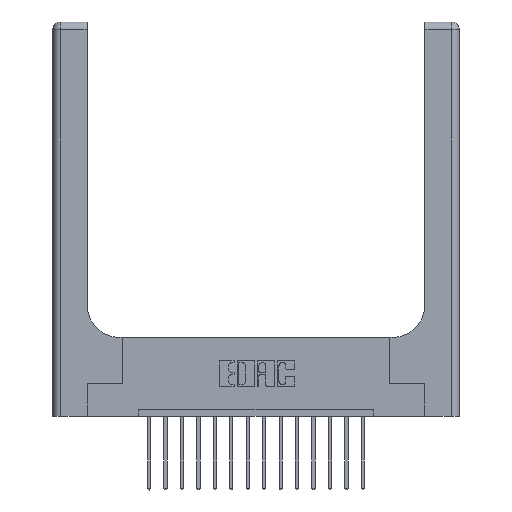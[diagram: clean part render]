
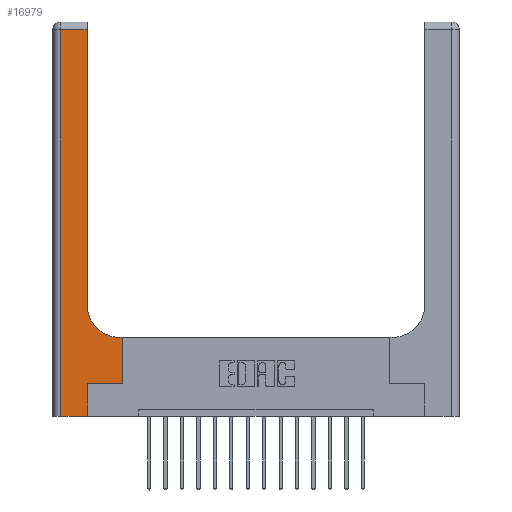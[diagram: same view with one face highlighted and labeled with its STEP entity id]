
A CAD part, top view. The second image highlights one B-rep face of the part: STEP entity #16979.
In plain terms, the highlighted planar face has unit normal (0, 0, 1).
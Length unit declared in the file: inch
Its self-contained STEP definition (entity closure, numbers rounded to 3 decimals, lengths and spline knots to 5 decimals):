
#4 = LINE ( 'NONE', #4893, #426 ) ;
#426 = VECTOR ( 'NONE', #14502, 39.37008 ) ;
#449 = VECTOR ( 'NONE', #7445, 39.37008 ) ;
#669 = EDGE_LOOP ( 'NONE', ( #3771, #2051, #6444, #8317, #9738, #2383, #13014, #2605, #9213 ) ) ;
#697 = DIRECTION ( 'NONE',  ( 0., 1., 0. ) ) ;
#824 = CARTESIAN_POINT ( 'NONE',  ( 0.26, 0.85, 0.37 ) ) ;
#1554 = CARTESIAN_POINT ( 'NONE',  ( 0.265, 0.25, 0.37 ) ) ;
#1566 = EDGE_CURVE ( 'NONE', #2639, #10057, #16916, .T. ) ;
#1581 = VECTOR ( 'NONE', #7155, 39.37008 ) ;
#1638 = LINE ( 'NONE', #5879, #2692 ) ;
#1983 = VECTOR ( 'NONE', #6688, 39.37008 ) ;
#2051 = ORIENTED_EDGE ( 'NONE', *, *, #12430, .T. ) ;
#2168 = VERTEX_POINT ( 'NONE', #14640 ) ;
#2310 = CARTESIAN_POINT ( 'NONE',  ( 0., 3., 0.37 ) ) ;
#2383 = ORIENTED_EDGE ( 'NONE', *, *, #7090, .T. ) ;
#2605 = ORIENTED_EDGE ( 'NONE', *, *, #15315, .T. ) ;
#2639 = VERTEX_POINT ( 'NONE', #14364 ) ;
#2692 = VECTOR ( 'NONE', #697, 39.37008 ) ;
#2784 = LINE ( 'NONE', #7039, #449 ) ;
#2826 = VERTEX_POINT ( 'NONE', #6256 ) ;
#2835 = CARTESIAN_POINT ( 'NONE',  ( 0.265, 0., 0.37 ) ) ;
#2977 = DIRECTION ( 'NONE',  ( 1., 0., 0. ) ) ;
#3338 = DIRECTION ( 'NONE',  ( 0., -1., 0. ) ) ;
#3771 = ORIENTED_EDGE ( 'NONE', *, *, #7831, .T. ) ;
#3782 = DIRECTION ( 'NONE',  ( 0., 0., -1. ) ) ;
#3832 = CARTESIAN_POINT ( 'NONE',  ( 0.51, 0.85, 0.37 ) ) ;
#4893 = CARTESIAN_POINT ( 'NONE',  ( 0., 2.94, 0.37 ) ) ;
#5879 = CARTESIAN_POINT ( 'NONE',  ( 0.26, 3., 0.37 ) ) ;
#5932 = CARTESIAN_POINT ( 'NONE',  ( 0.528, 0.25, 0.37 ) ) ;
#6047 = FACE_OUTER_BOUND ( 'NONE', #669, .T. ) ;
#6256 = CARTESIAN_POINT ( 'NONE',  ( 0.528, 0.6, 0.37 ) ) ;
#6405 = DIRECTION ( 'NONE',  ( 0., 0., -1. ) ) ;
#6444 = ORIENTED_EDGE ( 'NONE', *, *, #16345, .T. ) ;
#6688 = DIRECTION ( 'NONE',  ( 0., 1., 0. ) ) ;
#6909 = VECTOR ( 'NONE', #3338, 39.37008 ) ;
#7039 = CARTESIAN_POINT ( 'NONE',  ( 0., 0., 0.37 ) ) ;
#7066 = DIRECTION ( 'NONE',  ( -1., 0., 0. ) ) ;
#7090 = EDGE_CURVE ( 'NONE', #14016, #17511, #9363, .T. ) ;
#7155 = DIRECTION ( 'NONE',  ( 0., 1., 0. ) ) ;
#7445 = DIRECTION ( 'NONE',  ( 1., 0., 0. ) ) ;
#7744 = LINE ( 'NONE', #11412, #6909 ) ;
#7831 = EDGE_CURVE ( 'NONE', #10057, #2168, #1638, .T. ) ;
#8189 = LINE ( 'NONE', #8544, #1581 ) ;
#8317 = ORIENTED_EDGE ( 'NONE', *, *, #11874, .T. ) ;
#8544 = CARTESIAN_POINT ( 'NONE',  ( 0.265, 0., 0.37 ) ) ;
#9213 = ORIENTED_EDGE ( 'NONE', *, *, #1566, .T. ) ;
#9327 = CARTESIAN_POINT ( 'NONE',  ( 0.06, 0., 0.37 ) ) ;
#9363 = LINE ( 'NONE', #1554, #14288 ) ;
#9738 = ORIENTED_EDGE ( 'NONE', *, *, #16176, .T. ) ;
#10057 = VERTEX_POINT ( 'NONE', #824 ) ;
#10317 = CARTESIAN_POINT ( 'NONE',  ( 0.265, 0.25, 0.37 ) ) ;
#10471 = EDGE_CURVE ( 'NONE', #17511, #2826, #13315, .T. ) ;
#11100 = AXIS2_PLACEMENT_3D ( 'NONE', #3832, #3782, #13354 ) ;
#11412 = CARTESIAN_POINT ( 'NONE',  ( 0.06, 3., 0.37 ) ) ;
#11871 = DIRECTION ( 'NONE',  ( -1., 0., 0. ) ) ;
#11874 = EDGE_CURVE ( 'NONE', #14666, #12196, #2784, .T. ) ;
#12196 = VERTEX_POINT ( 'NONE', #2835 ) ;
#12430 = EDGE_CURVE ( 'NONE', #2168, #15359, #4, .T. ) ;
#12743 = VECTOR ( 'NONE', #7066, 39.37008 ) ;
#13014 = ORIENTED_EDGE ( 'NONE', *, *, #10471, .T. ) ;
#13242 = PLANE ( 'NONE',  #15475 ) ;
#13315 = LINE ( 'NONE', #14660, #1983 ) ;
#13354 = DIRECTION ( 'NONE',  ( 1., 0., 0. ) ) ;
#14016 = VERTEX_POINT ( 'NONE', #10317 ) ;
#14288 = VECTOR ( 'NONE', #2977, 39.37008 ) ;
#14364 = CARTESIAN_POINT ( 'NONE',  ( 0.51, 0.6, 0.37 ) ) ;
#14502 = DIRECTION ( 'NONE',  ( -1., 0., 0. ) ) ;
#14640 = CARTESIAN_POINT ( 'NONE',  ( 0.26, 2.94, 0.37 ) ) ;
#14660 = CARTESIAN_POINT ( 'NONE',  ( 0.528, 0.25, 0.37 ) ) ;
#14666 = VERTEX_POINT ( 'NONE', #9327 ) ;
#15315 = EDGE_CURVE ( 'NONE', #2826, #2639, #16774, .T. ) ;
#15359 = VERTEX_POINT ( 'NONE', #15941 ) ;
#15475 = AXIS2_PLACEMENT_3D ( 'NONE', #2310, #6405, #11871 ) ;
#15941 = CARTESIAN_POINT ( 'NONE',  ( 0.06, 2.94, 0.37 ) ) ;
#16176 = EDGE_CURVE ( 'NONE', #12196, #14016, #8189, .T. ) ;
#16345 = EDGE_CURVE ( 'NONE', #15359, #14666, #7744, .T. ) ;
#16774 = LINE ( 'NONE', #17679, #12743 ) ;
#16916 = CIRCLE ( 'NONE', #11100, 0.25 ) ;
#16979 = ADVANCED_FACE ( 'NONE', ( #6047 ), #13242, .F. ) ;
#17511 = VERTEX_POINT ( 'NONE', #5932 ) ;
#17679 = CARTESIAN_POINT ( 'NONE',  ( 0.26, 0.6, 0.37 ) ) ;
